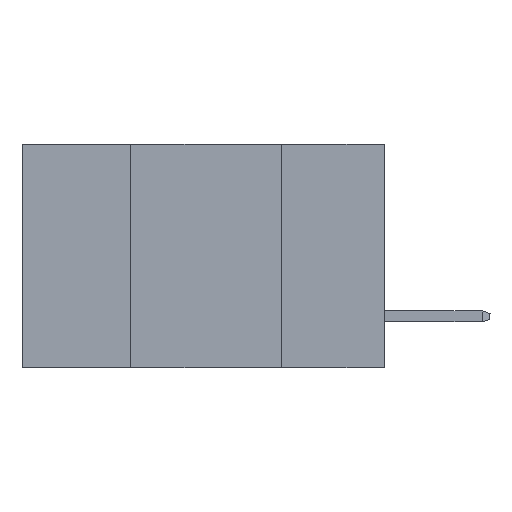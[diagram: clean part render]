
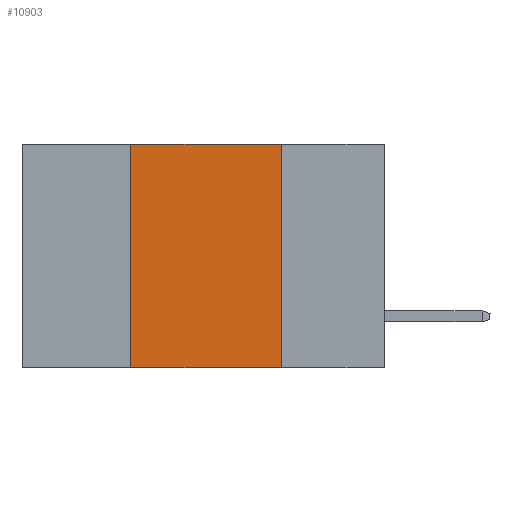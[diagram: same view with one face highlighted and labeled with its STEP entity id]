
A CAD part, left-side view. The second image highlights one B-rep face of the part: STEP entity #10903.
In plain terms, the highlighted planar face has unit normal (-1, 0, 0).
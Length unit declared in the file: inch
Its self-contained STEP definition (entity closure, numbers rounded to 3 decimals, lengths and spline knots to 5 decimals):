
#380 = CARTESIAN_POINT ( 'NONE',  ( 0., 0.17, -0.37 ) ) ;
#546 = CARTESIAN_POINT ( 'NONE',  ( 0., 0.6, 0. ) ) ;
#711 = VERTEX_POINT ( 'NONE', #11933 ) ;
#718 = PLANE ( 'NONE',  #7488 ) ;
#943 = CARTESIAN_POINT ( 'NONE',  ( 0., 0.6, 0. ) ) ;
#976 = VECTOR ( 'NONE', #11670, 39.37008 ) ;
#1099 = CARTESIAN_POINT ( 'NONE',  ( 0., 0.42, 0. ) ) ;
#1846 = DIRECTION ( 'NONE',  ( 0., 0., -1. ) ) ;
#2255 = ORIENTED_EDGE ( 'NONE', *, *, #2307, .T. ) ;
#2307 = EDGE_CURVE ( 'NONE', #8764, #3249, #10309, .T. ) ;
#2324 = CARTESIAN_POINT ( 'NONE',  ( 0., 0.6, -0.37 ) ) ;
#3073 = EDGE_LOOP ( 'NONE', ( #14647, #8984, #13500, #2255 ) ) ;
#3249 = VERTEX_POINT ( 'NONE', #380 ) ;
#3420 = VECTOR ( 'NONE', #6756, 39.37008 ) ;
#3495 = EDGE_CURVE ( 'NONE', #11725, #711, #7542, .T. ) ;
#4015 = CARTESIAN_POINT ( 'NONE',  ( 0., 0.42, -0.37 ) ) ;
#4133 = LINE ( 'NONE', #14558, #8691 ) ;
#4532 = LINE ( 'NONE', #10241, #3420 ) ;
#5100 = DIRECTION ( 'NONE',  ( 0., -1., 0. ) ) ;
#5349 = DIRECTION ( 'NONE',  ( 0., 0., -1. ) ) ;
#5446 = EDGE_CURVE ( 'NONE', #8764, #11725, #4532, .T. ) ;
#6600 = EDGE_CURVE ( 'NONE', #711, #3249, #4133, .T. ) ;
#6756 = DIRECTION ( 'NONE',  ( 0., 0., 1. ) ) ;
#7488 = AXIS2_PLACEMENT_3D ( 'NONE', #943, #9969, #5349 ) ;
#7542 = LINE ( 'NONE', #546, #13399 ) ;
#8691 = VECTOR ( 'NONE', #1846, 39.37008 ) ;
#8764 = VERTEX_POINT ( 'NONE', #4015 ) ;
#8984 = ORIENTED_EDGE ( 'NONE', *, *, #3495, .F. ) ;
#9969 = DIRECTION ( 'NONE',  ( 1., 0., 0. ) ) ;
#10241 = CARTESIAN_POINT ( 'NONE',  ( 0., 0.42, -0.37 ) ) ;
#10309 = LINE ( 'NONE', #2324, #976 ) ;
#10903 = ADVANCED_FACE ( 'NONE', ( #12513 ), #718, .F. ) ;
#11670 = DIRECTION ( 'NONE',  ( 0., -1., 0. ) ) ;
#11725 = VERTEX_POINT ( 'NONE', #1099 ) ;
#11933 = CARTESIAN_POINT ( 'NONE',  ( 0., 0.17, 0. ) ) ;
#12513 = FACE_OUTER_BOUND ( 'NONE', #3073, .T. ) ;
#13399 = VECTOR ( 'NONE', #5100, 39.37008 ) ;
#13500 = ORIENTED_EDGE ( 'NONE', *, *, #5446, .F. ) ;
#14558 = CARTESIAN_POINT ( 'NONE',  ( 0., 0.17, -0.37 ) ) ;
#14647 = ORIENTED_EDGE ( 'NONE', *, *, #6600, .F. ) ;
